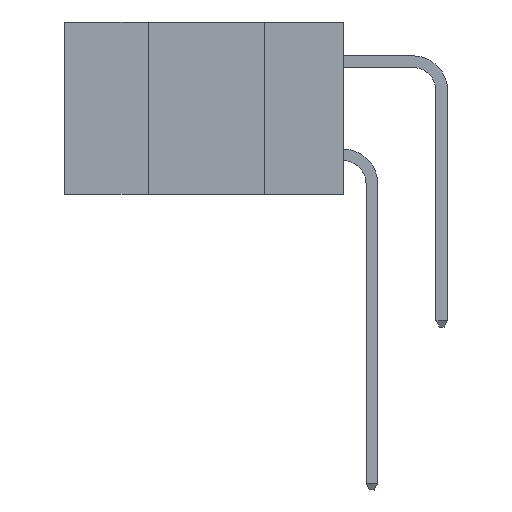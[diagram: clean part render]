
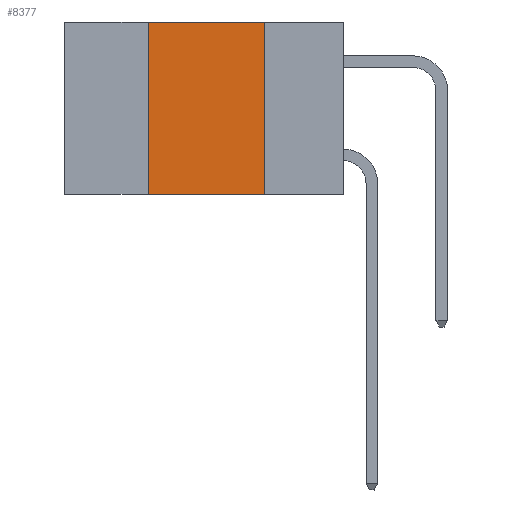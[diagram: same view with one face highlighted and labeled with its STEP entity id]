
A CAD part, left-side view. The second image highlights one B-rep face of the part: STEP entity #8377.
In plain terms, the highlighted planar face has unit normal (-1, 0, 0).
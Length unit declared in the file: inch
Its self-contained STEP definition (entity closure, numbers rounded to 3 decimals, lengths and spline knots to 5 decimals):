
#421 = CARTESIAN_POINT ( 'NONE',  ( 0., 0.6, -0.37 ) ) ;
#730 = DIRECTION ( 'NONE',  ( 0., -1., 0. ) ) ;
#1252 = PLANE ( 'NONE',  #9523 ) ;
#1325 = DIRECTION ( 'NONE',  ( 1., 0., 0. ) ) ;
#2484 = EDGE_CURVE ( 'NONE', #4619, #3365, #3462, .T. ) ;
#2872 = DIRECTION ( 'NONE',  ( 0., 0., -1. ) ) ;
#2950 = CARTESIAN_POINT ( 'NONE',  ( 0., 0.17, 0. ) ) ;
#2971 = CARTESIAN_POINT ( 'NONE',  ( 0., 0.6, 0. ) ) ;
#2975 = CARTESIAN_POINT ( 'NONE',  ( 0., 0.17, -0.37 ) ) ;
#3365 = VERTEX_POINT ( 'NONE', #2975 ) ;
#3462 = LINE ( 'NONE', #421, #19582 ) ;
#4364 = CARTESIAN_POINT ( 'NONE',  ( 0., 0.42, 0. ) ) ;
#4619 = VERTEX_POINT ( 'NONE', #13964 ) ;
#6217 = ORIENTED_EDGE ( 'NONE', *, *, #15063, .F. ) ;
#6320 = CARTESIAN_POINT ( 'NONE',  ( 0., 0.17, 0. ) ) ;
#6837 = VECTOR ( 'NONE', #2872, 39.37008 ) ;
#7088 = LINE ( 'NONE', #2950, #6837 ) ;
#7322 = VECTOR ( 'NONE', #15809, 39.37008 ) ;
#7764 = VECTOR ( 'NONE', #13121, 39.37008 ) ;
#7915 = CARTESIAN_POINT ( 'NONE',  ( 0., 0.6, 0. ) ) ;
#8377 = ADVANCED_FACE ( 'NONE', ( #11259 ), #1252, .F. ) ;
#9523 = AXIS2_PLACEMENT_3D ( 'NONE', #2971, #1325, #21585 ) ;
#11064 = ORIENTED_EDGE ( 'NONE', *, *, #12873, .F. ) ;
#11259 = FACE_OUTER_BOUND ( 'NONE', #14114, .T. ) ;
#12873 = EDGE_CURVE ( 'NONE', #4619, #17478, #18361, .T. ) ;
#13121 = DIRECTION ( 'NONE',  ( 0., -1., 0. ) ) ;
#13910 = ORIENTED_EDGE ( 'NONE', *, *, #20756, .F. ) ;
#13964 = CARTESIAN_POINT ( 'NONE',  ( 0., 0.42, -0.37 ) ) ;
#14114 = EDGE_LOOP ( 'NONE', ( #13910, #6217, #11064, #16524 ) ) ;
#14848 = CARTESIAN_POINT ( 'NONE',  ( 0., 0.42, 0. ) ) ;
#15063 = EDGE_CURVE ( 'NONE', #17478, #18327, #21773, .T. ) ;
#15809 = DIRECTION ( 'NONE',  ( 0., 0., 1. ) ) ;
#16524 = ORIENTED_EDGE ( 'NONE', *, *, #2484, .T. ) ;
#17478 = VERTEX_POINT ( 'NONE', #4364 ) ;
#18327 = VERTEX_POINT ( 'NONE', #6320 ) ;
#18361 = LINE ( 'NONE', #14848, #7322 ) ;
#19582 = VECTOR ( 'NONE', #730, 39.37008 ) ;
#20756 = EDGE_CURVE ( 'NONE', #18327, #3365, #7088, .T. ) ;
#21585 = DIRECTION ( 'NONE',  ( 0., 0., -1. ) ) ;
#21773 = LINE ( 'NONE', #7915, #7764 ) ;
